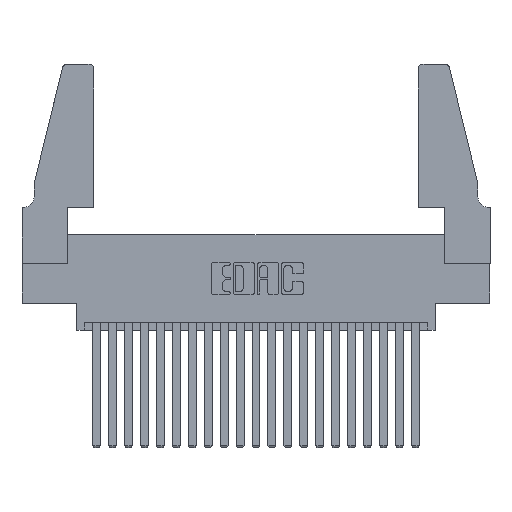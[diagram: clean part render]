
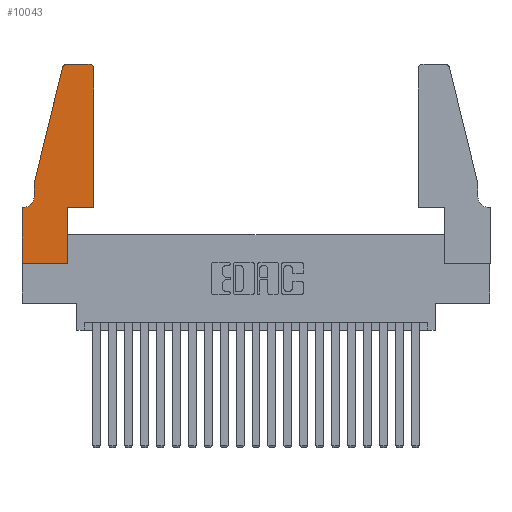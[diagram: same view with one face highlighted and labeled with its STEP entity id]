
A CAD part, top view. The second image highlights one B-rep face of the part: STEP entity #10043.
In plain terms, the highlighted planar face has unit normal (0, 0, 1).
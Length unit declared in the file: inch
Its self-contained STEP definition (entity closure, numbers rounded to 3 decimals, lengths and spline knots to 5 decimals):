
#65 = LINE ( 'NONE', #4078, #11971 ) ;
#539 = VECTOR ( 'NONE', #10657, 39.37008 ) ;
#820 = DIRECTION ( 'NONE',  ( 0., -1., 0. ) ) ;
#951 = ORIENTED_EDGE ( 'NONE', *, *, #19005, .T. ) ;
#1138 = VERTEX_POINT ( 'NONE', #8375 ) ;
#1337 = CARTESIAN_POINT ( 'NONE',  ( 0.4205, 1.22, 0.37 ) ) ;
#1442 = VERTEX_POINT ( 'NONE', #19398 ) ;
#1536 = CARTESIAN_POINT ( 'NONE',  ( 0.2605, 1.25, 0.37 ) ) ;
#1602 = DIRECTION ( 'NONE',  ( 0., 1., 0. ) ) ;
#1823 = EDGE_CURVE ( 'NONE', #14401, #12121, #2366, .T. ) ;
#1960 = AXIS2_PLACEMENT_3D ( 'NONE', #3779, #13581, #5222 ) ;
#2193 = LINE ( 'NONE', #10672, #18761 ) ;
#2366 = LINE ( 'NONE', #10309, #19441 ) ;
#2891 = VERTEX_POINT ( 'NONE', #10323 ) ;
#2960 = DIRECTION ( 'NONE',  ( 0., 0., 1. ) ) ;
#3097 = DIRECTION ( 'NONE',  ( -1., 0., 0. ) ) ;
#3340 = LINE ( 'NONE', #14324, #14489 ) ;
#3477 = EDGE_CURVE ( 'NONE', #14287, #2891, #20414, .T. ) ;
#3542 = LINE ( 'NONE', #15378, #7242 ) ;
#3779 = CARTESIAN_POINT ( 'NONE',  ( 0.284, 1.22, 0.37 ) ) ;
#4059 = ORIENTED_EDGE ( 'NONE', *, *, #14621, .T. ) ;
#4078 = CARTESIAN_POINT ( 'NONE',  ( 0., 0., 0.37 ) ) ;
#5010 = CARTESIAN_POINT ( 'NONE',  ( 0., 0.35, 0.37 ) ) ;
#5027 = DIRECTION ( 'NONE',  ( -1., 0., 0. ) ) ;
#5142 = ORIENTED_EDGE ( 'NONE', *, *, #15027, .T. ) ;
#5222 = DIRECTION ( 'NONE',  ( 1., 0., 0. ) ) ;
#5318 = ORIENTED_EDGE ( 'NONE', *, *, #13256, .T. ) ;
#5628 = LINE ( 'NONE', #11140, #14936 ) ;
#5695 = CARTESIAN_POINT ( 'NONE',  ( 0.25487, 1.22718, 0.37 ) ) ;
#5698 = VECTOR ( 'NONE', #6168, 39.37008 ) ;
#6168 = DIRECTION ( 'NONE',  ( 0., -1., 0. ) ) ;
#6430 = CARTESIAN_POINT ( 'NONE',  ( 0.284, 1.25, 0.37 ) ) ;
#6568 = AXIS2_PLACEMENT_3D ( 'NONE', #14956, #18274, #3097 ) ;
#6693 = CARTESIAN_POINT ( 'NONE',  ( 0.0755, 0.42, 0.37 ) ) ;
#7242 = VECTOR ( 'NONE', #1602, 39.37008 ) ;
#7821 = CARTESIAN_POINT ( 'NONE',  ( 0.2865, 0., 0.37 ) ) ;
#7886 = VERTEX_POINT ( 'NONE', #15335 ) ;
#8313 = LINE ( 'NONE', #18757, #539 ) ;
#8375 = CARTESIAN_POINT ( 'NONE',  ( 0., 0.35, 0.37 ) ) ;
#8896 = DIRECTION ( 'NONE',  ( 0., 0., 1. ) ) ;
#9489 = DIRECTION ( 'NONE',  ( -1., 0., 0. ) ) ;
#10043 = ADVANCED_FACE ( 'NONE', ( #18080 ), #15150, .T. ) ;
#10054 = LINE ( 'NONE', #1536, #15981 ) ;
#10309 = CARTESIAN_POINT ( 'NONE',  ( 0.0755, 0.5, 0.37 ) ) ;
#10323 = CARTESIAN_POINT ( 'NONE',  ( 0.4205, 1.25, 0.37 ) ) ;
#10494 = VERTEX_POINT ( 'NONE', #6693 ) ;
#10544 = EDGE_CURVE ( 'NONE', #20208, #14287, #3542, .T. ) ;
#10631 = LINE ( 'NONE', #14250, #5698 ) ;
#10657 = DIRECTION ( 'NONE',  ( 0., 1., 0. ) ) ;
#10672 = CARTESIAN_POINT ( 'NONE',  ( 0., 0., 0.37 ) ) ;
#10918 = ORIENTED_EDGE ( 'NONE', *, *, #15874, .T. ) ;
#10973 = ORIENTED_EDGE ( 'NONE', *, *, #15997, .T. ) ;
#11101 = DIRECTION ( 'NONE',  ( 1., 0., 0. ) ) ;
#11117 = EDGE_CURVE ( 'NONE', #15489, #20208, #5628, .T. ) ;
#11140 = CARTESIAN_POINT ( 'NONE',  ( 0.4505, 0.35, 0.37 ) ) ;
#11159 = ORIENTED_EDGE ( 'NONE', *, *, #3477, .T. ) ;
#11695 = DIRECTION ( 'NONE',  ( 1., 0., 0. ) ) ;
#11768 = AXIS2_PLACEMENT_3D ( 'NONE', #5010, #8896, #17017 ) ;
#11971 = VECTOR ( 'NONE', #11695, 39.37008 ) ;
#12007 = AXIS2_PLACEMENT_3D ( 'NONE', #1337, #2960, #11101 ) ;
#12121 = VERTEX_POINT ( 'NONE', #18724 ) ;
#13239 = CIRCLE ( 'NONE', #1960, 0.03 ) ;
#13256 = EDGE_CURVE ( 'NONE', #1442, #19242, #65, .T. ) ;
#13427 = CARTESIAN_POINT ( 'NONE',  ( 0.4505, 0.35, 0.37 ) ) ;
#13581 = DIRECTION ( 'NONE',  ( 0., 0., 1. ) ) ;
#13636 = ORIENTED_EDGE ( 'NONE', *, *, #20573, .T. ) ;
#13909 = ORIENTED_EDGE ( 'NONE', *, *, #20571, .T. ) ;
#14250 = CARTESIAN_POINT ( 'NONE',  ( 0.0755, 0.5, 0.37 ) ) ;
#14287 = VERTEX_POINT ( 'NONE', #21382 ) ;
#14324 = CARTESIAN_POINT ( 'NONE',  ( 0.0755, 0.35, 0.37 ) ) ;
#14401 = VERTEX_POINT ( 'NONE', #5695 ) ;
#14489 = VECTOR ( 'NONE', #9489, 39.37008 ) ;
#14621 = EDGE_CURVE ( 'NONE', #19242, #15489, #8313, .T. ) ;
#14936 = VECTOR ( 'NONE', #15419, 39.37008 ) ;
#14956 = CARTESIAN_POINT ( 'NONE',  ( 0.0055, 0.42, 0.37 ) ) ;
#15027 = EDGE_CURVE ( 'NONE', #16622, #14401, #13239, .T. ) ;
#15150 = PLANE ( 'NONE',  #11768 ) ;
#15335 = CARTESIAN_POINT ( 'NONE',  ( 0.0055, 0.35, 0.37 ) ) ;
#15378 = CARTESIAN_POINT ( 'NONE',  ( 0.4505, 0.35, 0.37 ) ) ;
#15419 = DIRECTION ( 'NONE',  ( 1., 0., 0. ) ) ;
#15445 = CIRCLE ( 'NONE', #6568, 0.07 ) ;
#15489 = VERTEX_POINT ( 'NONE', #18909 ) ;
#15874 = EDGE_CURVE ( 'NONE', #2891, #16622, #10054, .T. ) ;
#15981 = VECTOR ( 'NONE', #5027, 39.37008 ) ;
#15997 = EDGE_CURVE ( 'NONE', #10494, #7886, #15445, .T. ) ;
#16622 = VERTEX_POINT ( 'NONE', #6430 ) ;
#16996 = DIRECTION ( 'NONE',  ( -0.239, -0.971, 0. ) ) ;
#17017 = DIRECTION ( 'NONE',  ( 1., 0., 0. ) ) ;
#18080 = FACE_OUTER_BOUND ( 'NONE', #20169, .T. ) ;
#18181 = ORIENTED_EDGE ( 'NONE', *, *, #10544, .T. ) ;
#18274 = DIRECTION ( 'NONE',  ( 0., 0., -1. ) ) ;
#18724 = CARTESIAN_POINT ( 'NONE',  ( 0.0755, 0.5, 0.37 ) ) ;
#18757 = CARTESIAN_POINT ( 'NONE',  ( 0.2865, 0.35, 0.37 ) ) ;
#18761 = VECTOR ( 'NONE', #820, 39.37008 ) ;
#18909 = CARTESIAN_POINT ( 'NONE',  ( 0.2865, 0.35, 0.37 ) ) ;
#19005 = EDGE_CURVE ( 'NONE', #1138, #1442, #2193, .T. ) ;
#19196 = ORIENTED_EDGE ( 'NONE', *, *, #1823, .T. ) ;
#19242 = VERTEX_POINT ( 'NONE', #7821 ) ;
#19398 = CARTESIAN_POINT ( 'NONE',  ( 0., 0., 0.37 ) ) ;
#19441 = VECTOR ( 'NONE', #16996, 39.37008 ) ;
#20169 = EDGE_LOOP ( 'NONE', ( #10918, #5142, #19196, #13909, #10973, #13636, #951, #5318, #4059, #20782, #18181, #11159 ) ) ;
#20208 = VERTEX_POINT ( 'NONE', #13427 ) ;
#20414 = CIRCLE ( 'NONE', #12007, 0.03 ) ;
#20571 = EDGE_CURVE ( 'NONE', #12121, #10494, #10631, .T. ) ;
#20573 = EDGE_CURVE ( 'NONE', #7886, #1138, #3340, .T. ) ;
#20782 = ORIENTED_EDGE ( 'NONE', *, *, #11117, .T. ) ;
#21382 = CARTESIAN_POINT ( 'NONE',  ( 0.4505, 1.22, 0.37 ) ) ;
